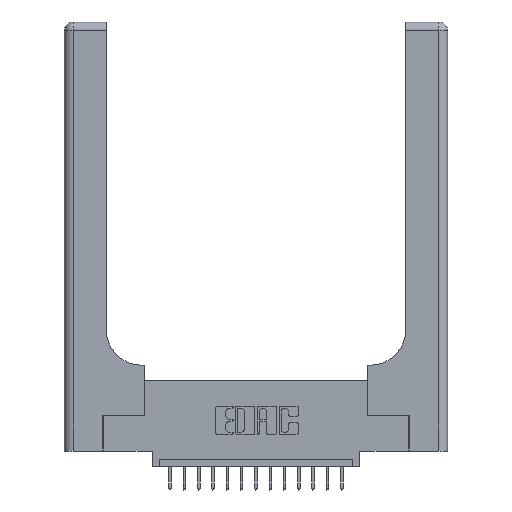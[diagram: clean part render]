
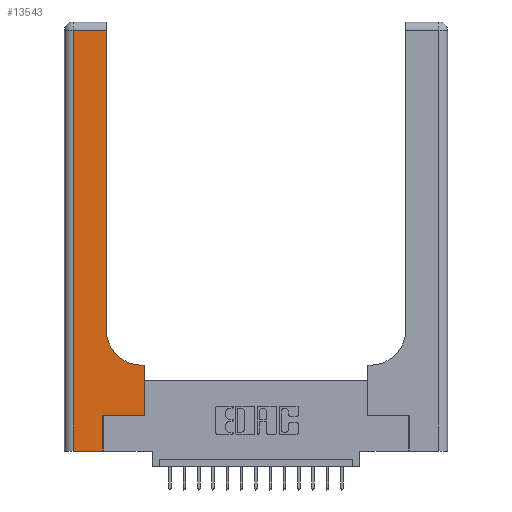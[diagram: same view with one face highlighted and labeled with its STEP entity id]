
A CAD part, top view. The second image highlights one B-rep face of the part: STEP entity #13543.
In plain terms, the highlighted planar face has unit normal (0, 0, 1).
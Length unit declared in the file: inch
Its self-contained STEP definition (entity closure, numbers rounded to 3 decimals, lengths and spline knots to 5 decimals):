
#37 = CARTESIAN_POINT ( 'NONE',  ( 0.06, 3., 0.37 ) ) ;
#261 = VECTOR ( 'NONE', #12005, 39.37008 ) ;
#387 = CARTESIAN_POINT ( 'NONE',  ( 0.5415, 0.6, 0.37 ) ) ;
#507 = VERTEX_POINT ( 'NONE', #18611 ) ;
#565 = ORIENTED_EDGE ( 'NONE', *, *, #2821, .T. ) ;
#769 = CARTESIAN_POINT ( 'NONE',  ( 0.06, 2.94, 0.37 ) ) ;
#1100 = ORIENTED_EDGE ( 'NONE', *, *, #14174, .T. ) ;
#1524 = ORIENTED_EDGE ( 'NONE', *, *, #12803, .T. ) ;
#1790 = DIRECTION ( 'NONE',  ( 0., 1., 0. ) ) ;
#1816 = EDGE_LOOP ( 'NONE', ( #1100, #565, #17481, #17677, #5074, #1524, #4793, #2384, #17918 ) ) ;
#2292 = EDGE_CURVE ( 'NONE', #2756, #2303, #15050, .T. ) ;
#2303 = VERTEX_POINT ( 'NONE', #387 ) ;
#2384 = ORIENTED_EDGE ( 'NONE', *, *, #2292, .T. ) ;
#2756 = VERTEX_POINT ( 'NONE', #7150 ) ;
#2821 = EDGE_CURVE ( 'NONE', #4412, #17211, #10417, .T. ) ;
#2918 = CARTESIAN_POINT ( 'NONE',  ( 0., 2.94, 0.37 ) ) ;
#3114 = VECTOR ( 'NONE', #13851, 39.37008 ) ;
#3271 = CARTESIAN_POINT ( 'NONE',  ( 0.5585, 0.25, 0.37 ) ) ;
#4024 = DIRECTION ( 'NONE',  ( 0., 0., -1. ) ) ;
#4252 = VECTOR ( 'NONE', #10188, 39.37008 ) ;
#4316 = CIRCLE ( 'NONE', #13731, 0.25 ) ;
#4412 = VERTEX_POINT ( 'NONE', #11101 ) ;
#4585 = CARTESIAN_POINT ( 'NONE',  ( 0.2915, 0.6, 0.37 ) ) ;
#4727 = CARTESIAN_POINT ( 'NONE',  ( 0.2915, 3., 0.37 ) ) ;
#4793 = ORIENTED_EDGE ( 'NONE', *, *, #5452, .T. ) ;
#4807 = VECTOR ( 'NONE', #6378, 39.37008 ) ;
#5026 = DIRECTION ( 'NONE',  ( 0., 0., -1. ) ) ;
#5074 = ORIENTED_EDGE ( 'NONE', *, *, #16265, .T. ) ;
#5424 = VECTOR ( 'NONE', #16335, 39.37008 ) ;
#5452 = EDGE_CURVE ( 'NONE', #8609, #2756, #6177, .T. ) ;
#5499 = VECTOR ( 'NONE', #17446, 39.37008 ) ;
#5752 = CARTESIAN_POINT ( 'NONE',  ( 0.06, 0., 0.37 ) ) ;
#5786 = EDGE_CURVE ( 'NONE', #13941, #13834, #14674, .T. ) ;
#6177 = LINE ( 'NONE', #6315, #4807 ) ;
#6315 = CARTESIAN_POINT ( 'NONE',  ( 0.5585, 0.25, 0.37 ) ) ;
#6378 = DIRECTION ( 'NONE',  ( 0., 1., 0. ) ) ;
#7150 = CARTESIAN_POINT ( 'NONE',  ( 0.5585, 0.6, 0.37 ) ) ;
#7917 = AXIS2_PLACEMENT_3D ( 'NONE', #17059, #4024, #15768 ) ;
#8175 = PLANE ( 'NONE',  #7917 ) ;
#8609 = VERTEX_POINT ( 'NONE', #3271 ) ;
#9839 = CARTESIAN_POINT ( 'NONE',  ( 0., 0., 0.37 ) ) ;
#10116 = DIRECTION ( 'NONE',  ( 0., -1., 0. ) ) ;
#10188 = DIRECTION ( 'NONE',  ( -1., 0., 0. ) ) ;
#10417 = LINE ( 'NONE', #2918, #4252 ) ;
#10829 = LINE ( 'NONE', #4727, #261 ) ;
#11101 = CARTESIAN_POINT ( 'NONE',  ( 0.2915, 2.94, 0.37 ) ) ;
#12005 = DIRECTION ( 'NONE',  ( 0., 1., 0. ) ) ;
#12046 = EDGE_CURVE ( 'NONE', #17211, #13941, #18769, .T. ) ;
#12803 = EDGE_CURVE ( 'NONE', #507, #8609, #14569, .T. ) ;
#13508 = CARTESIAN_POINT ( 'NONE',  ( 0.269, 0., 0.37 ) ) ;
#13543 = ADVANCED_FACE ( 'NONE', ( #13608 ), #8175, .F. ) ;
#13601 = CARTESIAN_POINT ( 'NONE',  ( 0.2915, 0.85, 0.37 ) ) ;
#13608 = FACE_OUTER_BOUND ( 'NONE', #1816, .T. ) ;
#13731 = AXIS2_PLACEMENT_3D ( 'NONE', #15421, #5026, #13920 ) ;
#13834 = VERTEX_POINT ( 'NONE', #18500 ) ;
#13851 = DIRECTION ( 'NONE',  ( 1., 0., 0. ) ) ;
#13920 = DIRECTION ( 'NONE',  ( 1., 0., 0. ) ) ;
#13941 = VERTEX_POINT ( 'NONE', #5752 ) ;
#14174 = EDGE_CURVE ( 'NONE', #18759, #4412, #10829, .T. ) ;
#14569 = LINE ( 'NONE', #15223, #3114 ) ;
#14674 = LINE ( 'NONE', #9839, #5499 ) ;
#15050 = LINE ( 'NONE', #4585, #5424 ) ;
#15223 = CARTESIAN_POINT ( 'NONE',  ( 0.269, 0.25, 0.37 ) ) ;
#15421 = CARTESIAN_POINT ( 'NONE',  ( 0.5415, 0.85, 0.37 ) ) ;
#15768 = DIRECTION ( 'NONE',  ( -1., 0., 0. ) ) ;
#16265 = EDGE_CURVE ( 'NONE', #13834, #507, #16989, .T. ) ;
#16335 = DIRECTION ( 'NONE',  ( -1., 0., 0. ) ) ;
#16989 = LINE ( 'NONE', #13508, #17444 ) ;
#17059 = CARTESIAN_POINT ( 'NONE',  ( 0., 3., 0.37 ) ) ;
#17203 = EDGE_CURVE ( 'NONE', #2303, #18759, #4316, .T. ) ;
#17211 = VERTEX_POINT ( 'NONE', #769 ) ;
#17444 = VECTOR ( 'NONE', #1790, 39.37008 ) ;
#17446 = DIRECTION ( 'NONE',  ( 1., 0., 0. ) ) ;
#17481 = ORIENTED_EDGE ( 'NONE', *, *, #12046, .T. ) ;
#17613 = VECTOR ( 'NONE', #10116, 39.37008 ) ;
#17677 = ORIENTED_EDGE ( 'NONE', *, *, #5786, .T. ) ;
#17918 = ORIENTED_EDGE ( 'NONE', *, *, #17203, .T. ) ;
#18500 = CARTESIAN_POINT ( 'NONE',  ( 0.269, 0., 0.37 ) ) ;
#18611 = CARTESIAN_POINT ( 'NONE',  ( 0.269, 0.25, 0.37 ) ) ;
#18759 = VERTEX_POINT ( 'NONE', #13601 ) ;
#18769 = LINE ( 'NONE', #37, #17613 ) ;
